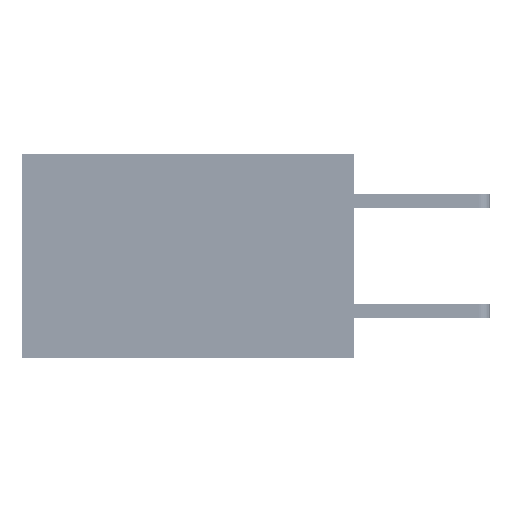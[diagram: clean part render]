
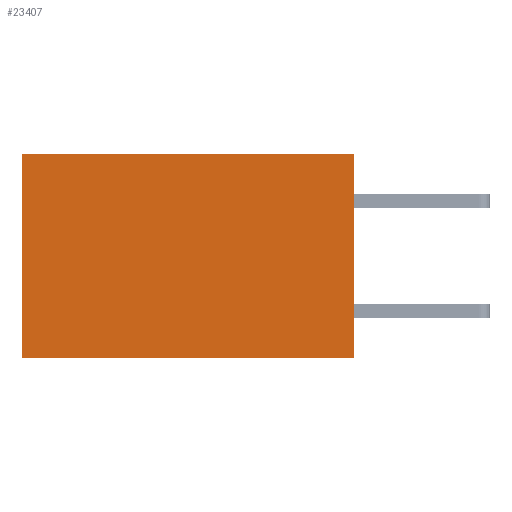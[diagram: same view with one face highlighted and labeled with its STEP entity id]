
A CAD part, left-side view. The second image highlights one B-rep face of the part: STEP entity #23407.
In plain terms, the highlighted planar face has unit normal (-1, 0, 0).
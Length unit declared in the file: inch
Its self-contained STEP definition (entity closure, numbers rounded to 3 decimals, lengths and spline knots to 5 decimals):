
#1471 = VERTEX_POINT ( 'NONE', #24438 ) ;
#4726 = DIRECTION ( 'NONE',  ( 0., 0., -1. ) ) ;
#4874 = CARTESIAN_POINT ( 'NONE',  ( 0.2875, 0.6, 0. ) ) ;
#6123 = LINE ( 'NONE', #8787, #42551 ) ;
#6285 = ORIENTED_EDGE ( 'NONE', *, *, #35653, .F. ) ;
#8749 = FACE_OUTER_BOUND ( 'NONE', #21447, .T. ) ;
#8787 = CARTESIAN_POINT ( 'NONE',  ( 0.2875, 0., 0. ) ) ;
#9702 = EDGE_CURVE ( 'NONE', #1471, #18656, #26354, .T. ) ;
#10490 = ORIENTED_EDGE ( 'NONE', *, *, #9702, .F. ) ;
#12349 = EDGE_CURVE ( 'NONE', #31411, #18656, #31806, .T. ) ;
#14149 = VECTOR ( 'NONE', #4726, 39.37008 ) ;
#15404 = ORIENTED_EDGE ( 'NONE', *, *, #12349, .T. ) ;
#15815 = CARTESIAN_POINT ( 'NONE',  ( 0.2875, 0.6, 0. ) ) ;
#16929 = VERTEX_POINT ( 'NONE', #45297 ) ;
#18199 = CARTESIAN_POINT ( 'NONE',  ( 0.2875, 0., -0.37 ) ) ;
#18656 = VERTEX_POINT ( 'NONE', #20506 ) ;
#19358 = DIRECTION ( 'NONE',  ( 0., 0., -1. ) ) ;
#20008 = DIRECTION ( 'NONE',  ( 0., 1., 0. ) ) ;
#20506 = CARTESIAN_POINT ( 'NONE',  ( 0.2875, 0.6, -0.37 ) ) ;
#21447 = EDGE_LOOP ( 'NONE', ( #15404, #10490, #6285, #29624 ) ) ;
#23407 = ADVANCED_FACE ( 'NONE', ( #8749 ), #41212, .F. ) ;
#24438 = CARTESIAN_POINT ( 'NONE',  ( 0.2875, 0., -0.37 ) ) ;
#26354 = LINE ( 'NONE', #18199, #45021 ) ;
#27050 = DIRECTION ( 'NONE',  ( 1., 0., 0. ) ) ;
#29624 = ORIENTED_EDGE ( 'NONE', *, *, #39768, .T. ) ;
#30099 = VECTOR ( 'NONE', #20008, 39.37008 ) ;
#31411 = VERTEX_POINT ( 'NONE', #15815 ) ;
#31806 = LINE ( 'NONE', #4874, #14149 ) ;
#35653 = EDGE_CURVE ( 'NONE', #16929, #1471, #6123, .T. ) ;
#37673 = CARTESIAN_POINT ( 'NONE',  ( 0.2875, 0., 0. ) ) ;
#38509 = AXIS2_PLACEMENT_3D ( 'NONE', #37673, #27050, #44708 ) ;
#39768 = EDGE_CURVE ( 'NONE', #16929, #31411, #45437, .T. ) ;
#41212 = PLANE ( 'NONE',  #38509 ) ;
#42551 = VECTOR ( 'NONE', #19358, 39.37008 ) ;
#42616 = DIRECTION ( 'NONE',  ( 0., 1., 0. ) ) ;
#44568 = CARTESIAN_POINT ( 'NONE',  ( 0.2875, 0., 0. ) ) ;
#44708 = DIRECTION ( 'NONE',  ( 0., 0., -1. ) ) ;
#45021 = VECTOR ( 'NONE', #42616, 39.37008 ) ;
#45297 = CARTESIAN_POINT ( 'NONE',  ( 0.2875, 0., 0. ) ) ;
#45437 = LINE ( 'NONE', #44568, #30099 ) ;
